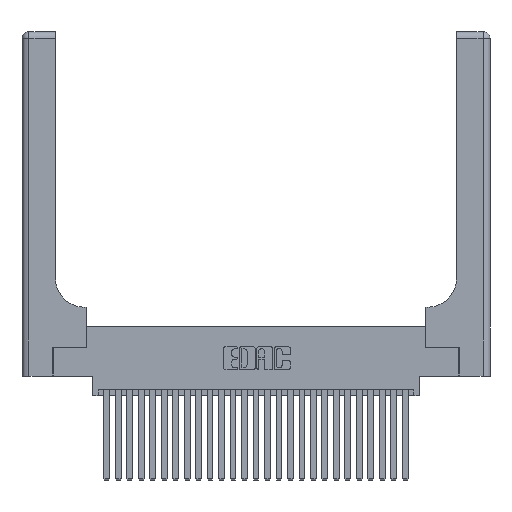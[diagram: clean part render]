
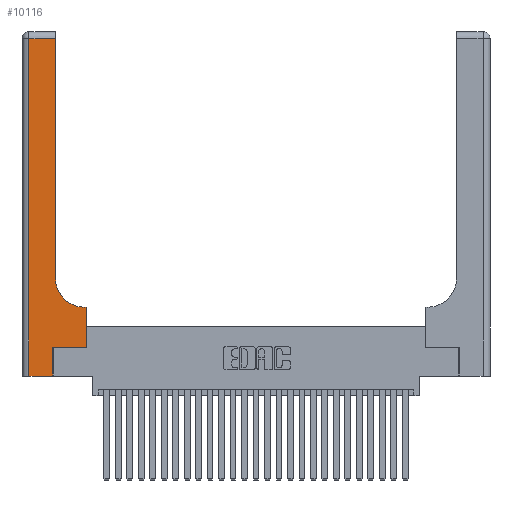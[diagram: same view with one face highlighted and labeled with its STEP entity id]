
A CAD part, top view. The second image highlights one B-rep face of the part: STEP entity #10116.
In plain terms, the highlighted planar face has unit normal (0, 0, 1).
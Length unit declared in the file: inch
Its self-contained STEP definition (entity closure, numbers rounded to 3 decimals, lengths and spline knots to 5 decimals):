
#114 = CARTESIAN_POINT ( 'NONE',  ( 0.2915, 0.85, 0.37 ) ) ;
#212 = CARTESIAN_POINT ( 'NONE',  ( 0.06, 0., 0.37 ) ) ;
#367 = VERTEX_POINT ( 'NONE', #8790 ) ;
#869 = LINE ( 'NONE', #5797, #1551 ) ;
#1433 = CARTESIAN_POINT ( 'NONE',  ( 0.5585, 0.25, 0.37 ) ) ;
#1551 = VECTOR ( 'NONE', #25473, 39.37008 ) ;
#1693 = EDGE_CURVE ( 'NONE', #8258, #367, #12229, .T. ) ;
#3046 = EDGE_LOOP ( 'NONE', ( #26716, #9274, #7365, #21040, #24350, #24651, #6235, #4626, #5389 ) ) ;
#4152 = EDGE_CURVE ( 'NONE', #7105, #18303, #4258, .T. ) ;
#4258 = CIRCLE ( 'NONE', #5039, 0.25 ) ;
#4434 = DIRECTION ( 'NONE',  ( 0., 1., 0. ) ) ;
#4626 = ORIENTED_EDGE ( 'NONE', *, *, #22527, .T. ) ;
#5039 = AXIS2_PLACEMENT_3D ( 'NONE', #26040, #19814, #6597 ) ;
#5291 = EDGE_CURVE ( 'NONE', #18303, #22427, #17931, .T. ) ;
#5389 = ORIENTED_EDGE ( 'NONE', *, *, #4152, .T. ) ;
#5797 = CARTESIAN_POINT ( 'NONE',  ( 0.269, 0., 0.37 ) ) ;
#6234 = LINE ( 'NONE', #8732, #20264 ) ;
#6235 = ORIENTED_EDGE ( 'NONE', *, *, #21277, .T. ) ;
#6441 = VERTEX_POINT ( 'NONE', #14982 ) ;
#6597 = DIRECTION ( 'NONE',  ( 1., 0., 0. ) ) ;
#6686 = CARTESIAN_POINT ( 'NONE',  ( 0.2915, 3., 0.37 ) ) ;
#7105 = VERTEX_POINT ( 'NONE', #18970 ) ;
#7304 = DIRECTION ( 'NONE',  ( -1., 0., 0. ) ) ;
#7365 = ORIENTED_EDGE ( 'NONE', *, *, #26814, .T. ) ;
#7410 = DIRECTION ( 'NONE',  ( 0., 0., -1. ) ) ;
#7903 = CARTESIAN_POINT ( 'NONE',  ( 0.269, 0.25, 0.37 ) ) ;
#8258 = VERTEX_POINT ( 'NONE', #212 ) ;
#8635 = AXIS2_PLACEMENT_3D ( 'NONE', #11805, #7410, #7304 ) ;
#8732 = CARTESIAN_POINT ( 'NONE',  ( 0.2915, 0.6, 0.37 ) ) ;
#8790 = CARTESIAN_POINT ( 'NONE',  ( 0.269, 0., 0.37 ) ) ;
#9045 = PLANE ( 'NONE',  #8635 ) ;
#9265 = DIRECTION ( 'NONE',  ( 1., 0., 0. ) ) ;
#9274 = ORIENTED_EDGE ( 'NONE', *, *, #9580, .T. ) ;
#9580 = EDGE_CURVE ( 'NONE', #22427, #6441, #24745, .T. ) ;
#9728 = CARTESIAN_POINT ( 'NONE',  ( 0., 2.94, 0.37 ) ) ;
#10116 = ADVANCED_FACE ( 'NONE', ( #15771 ), #9045, .F. ) ;
#10160 = DIRECTION ( 'NONE',  ( 0., -1., 0. ) ) ;
#11255 = VECTOR ( 'NONE', #9265, 39.37008 ) ;
#11591 = EDGE_CURVE ( 'NONE', #19690, #25022, #17764, .T. ) ;
#11805 = CARTESIAN_POINT ( 'NONE',  ( 0., 3., 0.37 ) ) ;
#12229 = LINE ( 'NONE', #14485, #17012 ) ;
#12274 = CARTESIAN_POINT ( 'NONE',  ( 0.269, 0.25, 0.37 ) ) ;
#14093 = VECTOR ( 'NONE', #4434, 39.37008 ) ;
#14485 = CARTESIAN_POINT ( 'NONE',  ( 0., 0., 0.37 ) ) ;
#14650 = CARTESIAN_POINT ( 'NONE',  ( 0.2915, 2.94, 0.37 ) ) ;
#14982 = CARTESIAN_POINT ( 'NONE',  ( 0.06, 2.94, 0.37 ) ) ;
#15166 = DIRECTION ( 'NONE',  ( 1., 0., 0. ) ) ;
#15771 = FACE_OUTER_BOUND ( 'NONE', #3046, .T. ) ;
#15954 = LINE ( 'NONE', #18928, #20048 ) ;
#16867 = VECTOR ( 'NONE', #26091, 39.37008 ) ;
#17012 = VECTOR ( 'NONE', #15166, 39.37008 ) ;
#17281 = EDGE_CURVE ( 'NONE', #367, #19690, #869, .T. ) ;
#17764 = LINE ( 'NONE', #12274, #11255 ) ;
#17931 = LINE ( 'NONE', #6686, #14093 ) ;
#18303 = VERTEX_POINT ( 'NONE', #114 ) ;
#18928 = CARTESIAN_POINT ( 'NONE',  ( 0.06, 3., 0.37 ) ) ;
#18970 = CARTESIAN_POINT ( 'NONE',  ( 0.5415, 0.6, 0.37 ) ) ;
#18977 = CARTESIAN_POINT ( 'NONE',  ( 0.5585, 0.6, 0.37 ) ) ;
#19463 = DIRECTION ( 'NONE',  ( -1., 0., 0. ) ) ;
#19690 = VERTEX_POINT ( 'NONE', #7903 ) ;
#19814 = DIRECTION ( 'NONE',  ( 0., 0., -1. ) ) ;
#20048 = VECTOR ( 'NONE', #10160, 39.37008 ) ;
#20264 = VECTOR ( 'NONE', #19463, 39.37008 ) ;
#21040 = ORIENTED_EDGE ( 'NONE', *, *, #1693, .T. ) ;
#21277 = EDGE_CURVE ( 'NONE', #25022, #22001, #21691, .T. ) ;
#21691 = LINE ( 'NONE', #1433, #22360 ) ;
#22001 = VERTEX_POINT ( 'NONE', #18977 ) ;
#22360 = VECTOR ( 'NONE', #25183, 39.37008 ) ;
#22427 = VERTEX_POINT ( 'NONE', #14650 ) ;
#22527 = EDGE_CURVE ( 'NONE', #22001, #7105, #6234, .T. ) ;
#24350 = ORIENTED_EDGE ( 'NONE', *, *, #17281, .T. ) ;
#24651 = ORIENTED_EDGE ( 'NONE', *, *, #11591, .T. ) ;
#24745 = LINE ( 'NONE', #9728, #16867 ) ;
#25022 = VERTEX_POINT ( 'NONE', #25973 ) ;
#25183 = DIRECTION ( 'NONE',  ( 0., 1., 0. ) ) ;
#25473 = DIRECTION ( 'NONE',  ( 0., 1., 0. ) ) ;
#25973 = CARTESIAN_POINT ( 'NONE',  ( 0.5585, 0.25, 0.37 ) ) ;
#26040 = CARTESIAN_POINT ( 'NONE',  ( 0.5415, 0.85, 0.37 ) ) ;
#26091 = DIRECTION ( 'NONE',  ( -1., 0., 0. ) ) ;
#26716 = ORIENTED_EDGE ( 'NONE', *, *, #5291, .T. ) ;
#26814 = EDGE_CURVE ( 'NONE', #6441, #8258, #15954, .T. ) ;
